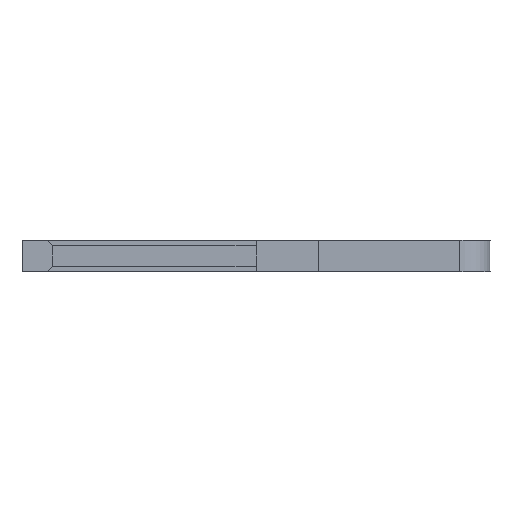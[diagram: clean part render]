
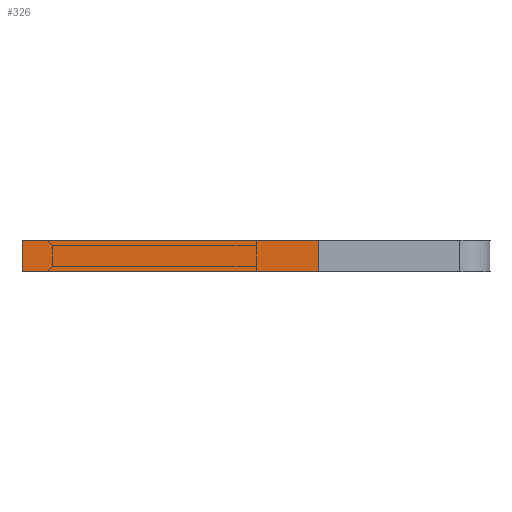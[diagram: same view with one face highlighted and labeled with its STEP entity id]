
A CAD part, left-side view. The second image highlights one B-rep face of the part: STEP entity #326.
In plain terms, the highlighted face is planar.
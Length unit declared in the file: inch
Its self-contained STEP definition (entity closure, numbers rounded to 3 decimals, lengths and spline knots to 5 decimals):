
#33 = CARTESIAN_POINT ( 'NONE',  ( -0.01, 0.15, -0.04 ) ) ;
#326 = ADVANCED_FACE ( 'NONE', ( #2187 ), #435, .F. ) ;
#431 = CARTESIAN_POINT ( 'NONE',  ( 0.01, 0.15, -0.04 ) ) ;
#435 = PLANE ( 'NONE',  #2459 ) ;
#447 = CARTESIAN_POINT ( 'NONE',  ( 0.01, 0.15, -0.04 ) ) ;
#586 = EDGE_CURVE ( 'NONE', #1072, #1096, #1672, .T. ) ;
#761 = DIRECTION ( 'NONE',  ( -1., 0., 0. ) ) ;
#840 = CARTESIAN_POINT ( 'NONE',  ( -0.01, 0.15, -0.04 ) ) ;
#925 = DIRECTION ( 'NONE',  ( -1., 0., 0. ) ) ;
#1016 = CARTESIAN_POINT ( 'NONE',  ( 0.01, 0.15, -0.04 ) ) ;
#1033 = VERTEX_POINT ( 'NONE', #1832 ) ;
#1072 = VERTEX_POINT ( 'NONE', #431 ) ;
#1096 = VERTEX_POINT ( 'NONE', #840 ) ;
#1336 = EDGE_LOOP ( 'NONE', ( #2001, #3552, #3058, #1938 ) ) ;
#1380 = VECTOR ( 'NONE', #2105, 39.37008 ) ;
#1392 = CARTESIAN_POINT ( 'NONE',  ( -0.01, -0.04, -0.04 ) ) ;
#1672 = LINE ( 'NONE', #447, #1813 ) ;
#1725 = VERTEX_POINT ( 'NONE', #1392 ) ;
#1813 = VECTOR ( 'NONE', #761, 39.37008 ) ;
#1832 = CARTESIAN_POINT ( 'NONE',  ( 0.01, -0.04, -0.04 ) ) ;
#1938 = ORIENTED_EDGE ( 'NONE', *, *, #3443, .T. ) ;
#2001 = ORIENTED_EDGE ( 'NONE', *, *, #3743, .T. ) ;
#2090 = VECTOR ( 'NONE', #3755, 39.37008 ) ;
#2098 = CARTESIAN_POINT ( 'NONE',  ( 0.01, 0.15, -0.04 ) ) ;
#2105 = DIRECTION ( 'NONE',  ( 0., 1., 0. ) ) ;
#2187 = FACE_OUTER_BOUND ( 'NONE', #1336, .T. ) ;
#2237 = DIRECTION ( 'NONE',  ( 0., 0., 1. ) ) ;
#2459 = AXIS2_PLACEMENT_3D ( 'NONE', #1016, #2237, #2860 ) ;
#2671 = LINE ( 'NONE', #33, #2090 ) ;
#2707 = EDGE_CURVE ( 'NONE', #1033, #1072, #2724, .T. ) ;
#2724 = LINE ( 'NONE', #2098, #1380 ) ;
#2768 = VECTOR ( 'NONE', #925, 39.37008 ) ;
#2860 = DIRECTION ( 'NONE',  ( 1., 0., 0. ) ) ;
#3058 = ORIENTED_EDGE ( 'NONE', *, *, #2707, .F. ) ;
#3390 = LINE ( 'NONE', #3682, #2768 ) ;
#3443 = EDGE_CURVE ( 'NONE', #1033, #1725, #3390, .T. ) ;
#3552 = ORIENTED_EDGE ( 'NONE', *, *, #586, .F. ) ;
#3682 = CARTESIAN_POINT ( 'NONE',  ( 0.01, -0.04, -0.04 ) ) ;
#3743 = EDGE_CURVE ( 'NONE', #1725, #1096, #2671, .T. ) ;
#3755 = DIRECTION ( 'NONE',  ( 0., 1., 0. ) ) ;
